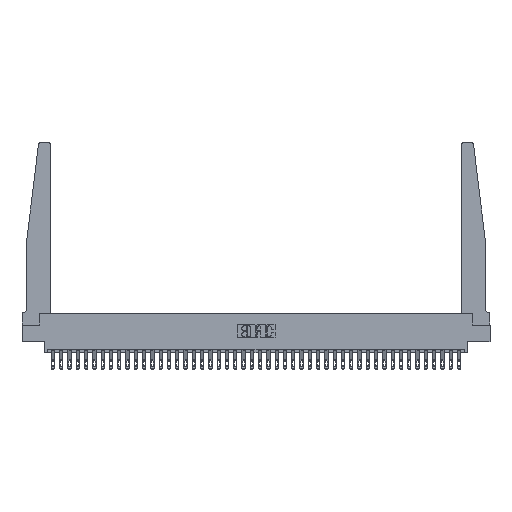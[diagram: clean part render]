
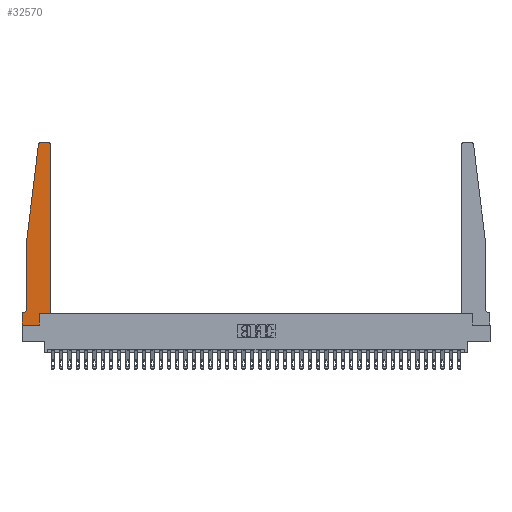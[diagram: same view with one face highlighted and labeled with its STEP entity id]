
A CAD part, top view. The second image highlights one B-rep face of the part: STEP entity #32570.
In plain terms, the highlighted planar face has unit normal (0, 0, 1).
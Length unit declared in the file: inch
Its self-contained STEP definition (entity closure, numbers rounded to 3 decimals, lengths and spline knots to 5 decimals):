
#120 = PLANE ( 'NONE',  #30683 ) ;
#507 = VERTEX_POINT ( 'NONE', #22940 ) ;
#858 = EDGE_LOOP ( 'NONE', ( #14415, #36040, #10773, #2226, #31631, #14806, #28957, #27172, #3590, #9410, #12137, #4499 ) ) ;
#1962 = VECTOR ( 'NONE', #2202, 39.37008 ) ;
#2202 = DIRECTION ( 'NONE',  ( -1., 0., 0. ) ) ;
#2226 = ORIENTED_EDGE ( 'NONE', *, *, #5713, .T. ) ;
#3094 = VERTEX_POINT ( 'NONE', #14150 ) ;
#3290 = FACE_OUTER_BOUND ( 'NONE', #858, .T. ) ;
#3366 = CARTESIAN_POINT ( 'NONE',  ( 0., 0., 0.37 ) ) ;
#3590 = ORIENTED_EDGE ( 'NONE', *, *, #35894, .T. ) ;
#4204 = CARTESIAN_POINT ( 'NONE',  ( 0.27653, 2.75, 0.37 ) ) ;
#4499 = ORIENTED_EDGE ( 'NONE', *, *, #31173, .T. ) ;
#4953 = LINE ( 'NONE', #6435, #26777 ) ;
#5441 = DIRECTION ( 'NONE',  ( 0., 1., 0. ) ) ;
#5450 = DIRECTION ( 'NONE',  ( 0., 0., -1. ) ) ;
#5542 = CARTESIAN_POINT ( 'NONE',  ( 0.395, 2.72, 0.37 ) ) ;
#5713 = EDGE_CURVE ( 'NONE', #3094, #507, #31708, .T. ) ;
#5908 = CARTESIAN_POINT ( 'NONE',  ( 0., 0.1875, 0.37 ) ) ;
#6087 = EDGE_CURVE ( 'NONE', #24880, #9703, #4953, .T. ) ;
#6435 = CARTESIAN_POINT ( 'NONE',  ( 0., 0., 0.37 ) ) ;
#6623 = LINE ( 'NONE', #15909, #36762 ) ;
#7694 = VECTOR ( 'NONE', #34399, 39.37008 ) ;
#8436 = DIRECTION ( 'NONE',  ( 1., 0., 0. ) ) ;
#8807 = DIRECTION ( 'NONE',  ( 1., 0., 0. ) ) ;
#9325 = DIRECTION ( 'NONE',  ( 1., 0., 0. ) ) ;
#9410 = ORIENTED_EDGE ( 'NONE', *, *, #19568, .T. ) ;
#9703 = VERTEX_POINT ( 'NONE', #35992 ) ;
#9707 = CARTESIAN_POINT ( 'NONE',  ( 0.015, 0.1875, 0.37 ) ) ;
#9855 = VECTOR ( 'NONE', #32346, 39.37008 ) ;
#10115 = DIRECTION ( 'NONE',  ( 0., 0., 1. ) ) ;
#10199 = VERTEX_POINT ( 'NONE', #4204 ) ;
#10233 = CIRCLE ( 'NONE', #27298, 0.03 ) ;
#10548 = CARTESIAN_POINT ( 'NONE',  ( 0.395, 2.75, 0.37 ) ) ;
#10666 = VECTOR ( 'NONE', #5441, 39.37008 ) ;
#10773 = ORIENTED_EDGE ( 'NONE', *, *, #25307, .T. ) ;
#10837 = CARTESIAN_POINT ( 'NONE',  ( 0., 0., 0.37 ) ) ;
#12043 = CIRCLE ( 'NONE', #33476, 0.03 ) ;
#12137 = ORIENTED_EDGE ( 'NONE', *, *, #24063, .T. ) ;
#12641 = CARTESIAN_POINT ( 'NONE',  ( 0.425, 0.18, 0.37 ) ) ;
#13018 = DIRECTION ( 'NONE',  ( -1., 0., 0. ) ) ;
#13521 = CARTESIAN_POINT ( 'NONE',  ( 0.24675, 2.72367, 0.37 ) ) ;
#13807 = CARTESIAN_POINT ( 'NONE',  ( 0.425, 0.18, 0.37 ) ) ;
#14150 = CARTESIAN_POINT ( 'NONE',  ( 0.065, 1.25, 0.37 ) ) ;
#14415 = ORIENTED_EDGE ( 'NONE', *, *, #29816, .T. ) ;
#14725 = DIRECTION ( 'NONE',  ( 1., 0., 0. ) ) ;
#14806 = ORIENTED_EDGE ( 'NONE', *, *, #20280, .T. ) ;
#15042 = VERTEX_POINT ( 'NONE', #9707 ) ;
#15322 = VERTEX_POINT ( 'NONE', #25073 ) ;
#15324 = VERTEX_POINT ( 'NONE', #13807 ) ;
#15647 = LINE ( 'NONE', #27150, #24042 ) ;
#15909 = CARTESIAN_POINT ( 'NONE',  ( 0.065, 1.25, 0.37 ) ) ;
#17657 = AXIS2_PLACEMENT_3D ( 'NONE', #22496, #5450, #25356 ) ;
#19568 = EDGE_CURVE ( 'NONE', #32762, #15324, #26993, .T. ) ;
#20280 = EDGE_CURVE ( 'NONE', #15042, #22383, #33116, .T. ) ;
#20967 = CARTESIAN_POINT ( 'NONE',  ( 0.2605, 0.18, 0.37 ) ) ;
#22377 = EDGE_CURVE ( 'NONE', #507, #15042, #33413, .T. ) ;
#22383 = VERTEX_POINT ( 'NONE', #36576 ) ;
#22496 = CARTESIAN_POINT ( 'NONE',  ( 0.015, 0.2375, 0.37 ) ) ;
#22831 = LINE ( 'NONE', #3366, #7694 ) ;
#22940 = CARTESIAN_POINT ( 'NONE',  ( 0.065, 0.2375, 0.37 ) ) ;
#23269 = VECTOR ( 'NONE', #24980, 39.37008 ) ;
#24042 = VECTOR ( 'NONE', #13018, 39.37008 ) ;
#24063 = EDGE_CURVE ( 'NONE', #15324, #15322, #24958, .T. ) ;
#24880 = VERTEX_POINT ( 'NONE', #10837 ) ;
#24958 = LINE ( 'NONE', #12641, #9855 ) ;
#24980 = DIRECTION ( 'NONE',  ( 0., -1., 0. ) ) ;
#25073 = CARTESIAN_POINT ( 'NONE',  ( 0.425, 2.72, 0.37 ) ) ;
#25307 = EDGE_CURVE ( 'NONE', #31695, #3094, #6623, .T. ) ;
#25356 = DIRECTION ( 'NONE',  ( -1., 0., 0. ) ) ;
#25443 = DIRECTION ( 'NONE',  ( 0., 0., 1. ) ) ;
#25812 = DIRECTION ( 'NONE',  ( 0., 0., 1. ) ) ;
#26777 = VECTOR ( 'NONE', #9325, 39.37008 ) ;
#26993 = LINE ( 'NONE', #28939, #34507 ) ;
#27104 = CARTESIAN_POINT ( 'NONE',  ( 0.27653, 2.72, 0.37 ) ) ;
#27150 = CARTESIAN_POINT ( 'NONE',  ( 0.25, 2.75, 0.37 ) ) ;
#27172 = ORIENTED_EDGE ( 'NONE', *, *, #6087, .T. ) ;
#27298 = AXIS2_PLACEMENT_3D ( 'NONE', #27104, #10115, #29958 ) ;
#28939 = CARTESIAN_POINT ( 'NONE',  ( 0.425, 0.18, 0.37 ) ) ;
#28957 = ORIENTED_EDGE ( 'NONE', *, *, #33319, .T. ) ;
#29118 = VERTEX_POINT ( 'NONE', #10548 ) ;
#29816 = EDGE_CURVE ( 'NONE', #29118, #10199, #15647, .T. ) ;
#29958 = DIRECTION ( 'NONE',  ( 1., 0., 0. ) ) ;
#30476 = EDGE_CURVE ( 'NONE', #10199, #31695, #10233, .T. ) ;
#30586 = CARTESIAN_POINT ( 'NONE',  ( 0.065, 0.1875, 0.37 ) ) ;
#30683 = AXIS2_PLACEMENT_3D ( 'NONE', #5908, #25812, #8807 ) ;
#31173 = EDGE_CURVE ( 'NONE', #15322, #29118, #12043, .T. ) ;
#31631 = ORIENTED_EDGE ( 'NONE', *, *, #22377, .T. ) ;
#31695 = VERTEX_POINT ( 'NONE', #13521 ) ;
#31708 = LINE ( 'NONE', #36191, #23269 ) ;
#32346 = DIRECTION ( 'NONE',  ( 0., 1., 0. ) ) ;
#32570 = ADVANCED_FACE ( 'NONE', ( #3290 ), #120, .T. ) ;
#32762 = VERTEX_POINT ( 'NONE', #20967 ) ;
#33116 = LINE ( 'NONE', #30586, #1962 ) ;
#33253 = LINE ( 'NONE', #36567, #10666 ) ;
#33319 = EDGE_CURVE ( 'NONE', #22383, #24880, #22831, .T. ) ;
#33413 = CIRCLE ( 'NONE', #17657, 0.05 ) ;
#33476 = AXIS2_PLACEMENT_3D ( 'NONE', #5542, #25443, #8436 ) ;
#34399 = DIRECTION ( 'NONE',  ( 0., -1., 0. ) ) ;
#34507 = VECTOR ( 'NONE', #14725, 39.37008 ) ;
#35666 = DIRECTION ( 'NONE',  ( -0.122, -0.992, 0. ) ) ;
#35894 = EDGE_CURVE ( 'NONE', #9703, #32762, #33253, .T. ) ;
#35992 = CARTESIAN_POINT ( 'NONE',  ( 0.2605, 0., 0.37 ) ) ;
#36040 = ORIENTED_EDGE ( 'NONE', *, *, #30476, .T. ) ;
#36191 = CARTESIAN_POINT ( 'NONE',  ( 0.065, 1.25, 0.37 ) ) ;
#36567 = CARTESIAN_POINT ( 'NONE',  ( 0.2605, 0.18, 0.37 ) ) ;
#36576 = CARTESIAN_POINT ( 'NONE',  ( 0., 0.1875, 0.37 ) ) ;
#36762 = VECTOR ( 'NONE', #35666, 39.37008 ) ;
